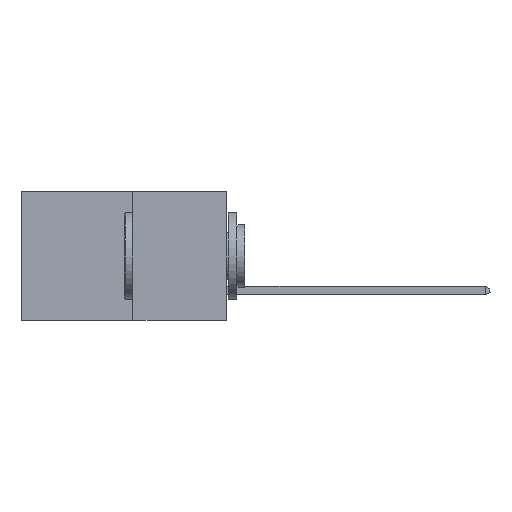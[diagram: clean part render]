
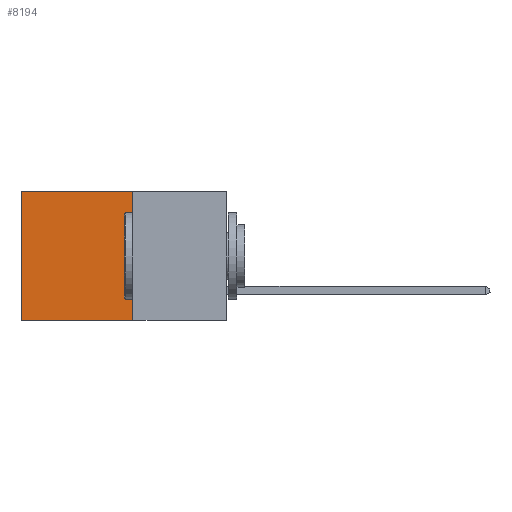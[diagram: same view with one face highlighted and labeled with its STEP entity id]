
A CAD part, left-side view. The second image highlights one B-rep face of the part: STEP entity #8194.
In plain terms, the highlighted planar face has unit normal (-1, 0, 0).
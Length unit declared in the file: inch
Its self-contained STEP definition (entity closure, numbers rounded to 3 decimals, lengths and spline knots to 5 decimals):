
#153 = EDGE_CURVE ( 'NONE', #5851, #3852, #4291, .T. ) ;
#607 = CARTESIAN_POINT ( 'NONE',  ( 0.277, 0.59, -0.37 ) ) ;
#2914 = VECTOR ( 'NONE', #19471, 39.37008 ) ;
#2989 = DIRECTION ( 'NONE',  ( 0., 1., 0. ) ) ;
#3706 = VERTEX_POINT ( 'NONE', #11318 ) ;
#3852 = VERTEX_POINT ( 'NONE', #6740 ) ;
#4291 = LINE ( 'NONE', #5432, #12010 ) ;
#4525 = CARTESIAN_POINT ( 'NONE',  ( 0.277, 0.27, -0.37 ) ) ;
#5091 = EDGE_CURVE ( 'NONE', #14858, #3706, #19568, .T. ) ;
#5384 = VECTOR ( 'NONE', #2989, 39.37008 ) ;
#5432 = CARTESIAN_POINT ( 'NONE',  ( 0.277, 0.27, -0.37 ) ) ;
#5851 = VERTEX_POINT ( 'NONE', #17967 ) ;
#6740 = CARTESIAN_POINT ( 'NONE',  ( 0.277, 0.27, -0.37 ) ) ;
#7022 = DIRECTION ( 'NONE',  ( 1., 0., 0. ) ) ;
#8194 = ADVANCED_FACE ( 'NONE', ( #11747 ), #11617, .F. ) ;
#8486 = ORIENTED_EDGE ( 'NONE', *, *, #5091, .T. ) ;
#8607 = ORIENTED_EDGE ( 'NONE', *, *, #17469, .F. ) ;
#8626 = ORIENTED_EDGE ( 'NONE', *, *, #153, .F. ) ;
#8695 = ORIENTED_EDGE ( 'NONE', *, *, #16392, .T. ) ;
#9322 = VECTOR ( 'NONE', #12325, 39.37008 ) ;
#10375 = DIRECTION ( 'NONE',  ( 0., 0., -1. ) ) ;
#11318 = CARTESIAN_POINT ( 'NONE',  ( 0.277, 0.59, -0.37 ) ) ;
#11546 = CARTESIAN_POINT ( 'NONE',  ( 0.277, 0.59, 0. ) ) ;
#11617 = PLANE ( 'NONE',  #13843 ) ;
#11747 = FACE_OUTER_BOUND ( 'NONE', #15227, .T. ) ;
#12010 = VECTOR ( 'NONE', #10375, 39.37008 ) ;
#12325 = DIRECTION ( 'NONE',  ( 0., 1., 0. ) ) ;
#13161 = CARTESIAN_POINT ( 'NONE',  ( 0.277, 0.27, -0.37 ) ) ;
#13841 = CARTESIAN_POINT ( 'NONE',  ( 0.277, 0.27, 0. ) ) ;
#13843 = AXIS2_PLACEMENT_3D ( 'NONE', #13161, #7022, #17709 ) ;
#14858 = VERTEX_POINT ( 'NONE', #11546 ) ;
#15227 = EDGE_LOOP ( 'NONE', ( #8486, #8607, #8626, #8695 ) ) ;
#16392 = EDGE_CURVE ( 'NONE', #5851, #14858, #17433, .T. ) ;
#17433 = LINE ( 'NONE', #13841, #9322 ) ;
#17469 = EDGE_CURVE ( 'NONE', #3852, #3706, #17557, .T. ) ;
#17557 = LINE ( 'NONE', #4525, #5384 ) ;
#17709 = DIRECTION ( 'NONE',  ( 0., 0., -1. ) ) ;
#17967 = CARTESIAN_POINT ( 'NONE',  ( 0.277, 0.27, 0. ) ) ;
#19471 = DIRECTION ( 'NONE',  ( 0., 0., -1. ) ) ;
#19568 = LINE ( 'NONE', #607, #2914 ) ;
